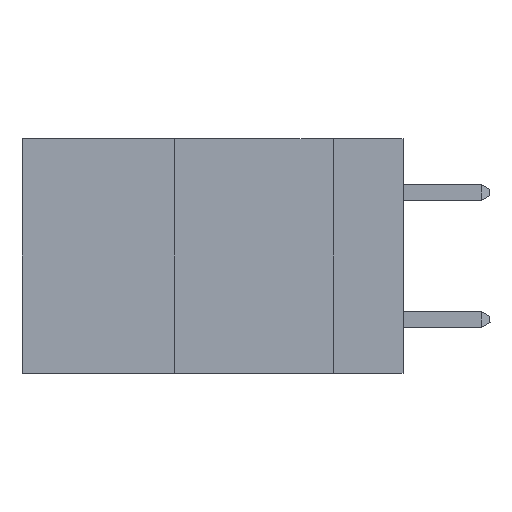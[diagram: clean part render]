
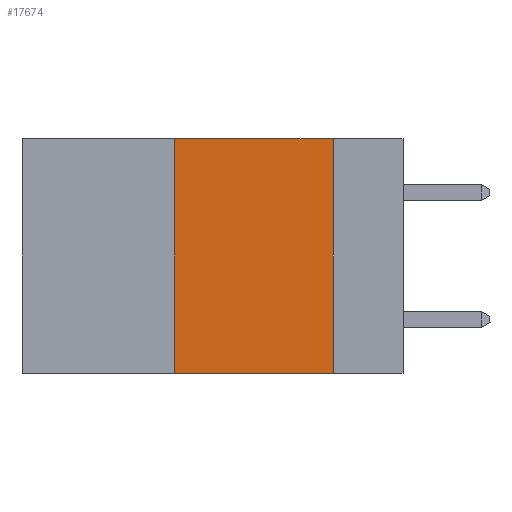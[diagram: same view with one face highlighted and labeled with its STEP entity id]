
A CAD part, left-side view. The second image highlights one B-rep face of the part: STEP entity #17674.
In plain terms, the highlighted planar face has unit normal (-1, 0, 0).
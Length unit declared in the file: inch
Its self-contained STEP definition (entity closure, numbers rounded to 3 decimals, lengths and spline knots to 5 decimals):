
#434 = LINE ( 'NONE', #6163, #41701 ) ;
#619 = VECTOR ( 'NONE', #7430, 39.37008 ) ;
#4181 = CARTESIAN_POINT ( 'NONE',  ( 0., 0.11, 0. ) ) ;
#6163 = CARTESIAN_POINT ( 'NONE',  ( 0., 0.36, 0. ) ) ;
#7430 = DIRECTION ( 'NONE',  ( 0., 0., -1. ) ) ;
#7478 = PLANE ( 'NONE',  #22564 ) ;
#7508 = EDGE_CURVE ( 'NONE', #19334, #14848, #31312, .T. ) ;
#7942 = CARTESIAN_POINT ( 'NONE',  ( 0., 0.6, 0. ) ) ;
#10027 = CARTESIAN_POINT ( 'NONE',  ( 0., 0.36, -0.37 ) ) ;
#12275 = EDGE_CURVE ( 'NONE', #41336, #19334, #26797, .T. ) ;
#14550 = DIRECTION ( 'NONE',  ( 0., 0., -1. ) ) ;
#14848 = VERTEX_POINT ( 'NONE', #37095 ) ;
#17022 = EDGE_CURVE ( 'NONE', #26406, #41336, #434, .T. ) ;
#17674 = ADVANCED_FACE ( 'NONE', ( #34397 ), #7478, .F. ) ;
#18434 = VECTOR ( 'NONE', #30518, 39.37008 ) ;
#19155 = ORIENTED_EDGE ( 'NONE', *, *, #17022, .F. ) ;
#19334 = VERTEX_POINT ( 'NONE', #43875 ) ;
#19513 = ORIENTED_EDGE ( 'NONE', *, *, #12275, .F. ) ;
#19600 = EDGE_LOOP ( 'NONE', ( #35505, #19513, #19155, #39614 ) ) ;
#22564 = AXIS2_PLACEMENT_3D ( 'NONE', #7942, #29201, #14550 ) ;
#26406 = VERTEX_POINT ( 'NONE', #10027 ) ;
#26797 = LINE ( 'NONE', #30219, #18434 ) ;
#29201 = DIRECTION ( 'NONE',  ( 1., 0., 0. ) ) ;
#30219 = CARTESIAN_POINT ( 'NONE',  ( 0., 0.6, 0. ) ) ;
#30518 = DIRECTION ( 'NONE',  ( 0., -1., 0. ) ) ;
#31312 = LINE ( 'NONE', #4181, #619 ) ;
#31523 = CARTESIAN_POINT ( 'NONE',  ( 0., 0.36, 0. ) ) ;
#31623 = DIRECTION ( 'NONE',  ( 0., -1., 0. ) ) ;
#34397 = FACE_OUTER_BOUND ( 'NONE', #19600, .T. ) ;
#34521 = LINE ( 'NONE', #45909, #37295 ) ;
#34741 = DIRECTION ( 'NONE',  ( 0., 0., 1. ) ) ;
#35505 = ORIENTED_EDGE ( 'NONE', *, *, #7508, .F. ) ;
#37095 = CARTESIAN_POINT ( 'NONE',  ( 0., 0.11, -0.37 ) ) ;
#37295 = VECTOR ( 'NONE', #31623, 39.37008 ) ;
#39614 = ORIENTED_EDGE ( 'NONE', *, *, #40433, .T. ) ;
#40433 = EDGE_CURVE ( 'NONE', #26406, #14848, #34521, .T. ) ;
#41336 = VERTEX_POINT ( 'NONE', #31523 ) ;
#41701 = VECTOR ( 'NONE', #34741, 39.37008 ) ;
#43875 = CARTESIAN_POINT ( 'NONE',  ( 0., 0.11, 0. ) ) ;
#45909 = CARTESIAN_POINT ( 'NONE',  ( 0., 0.6, -0.37 ) ) ;
